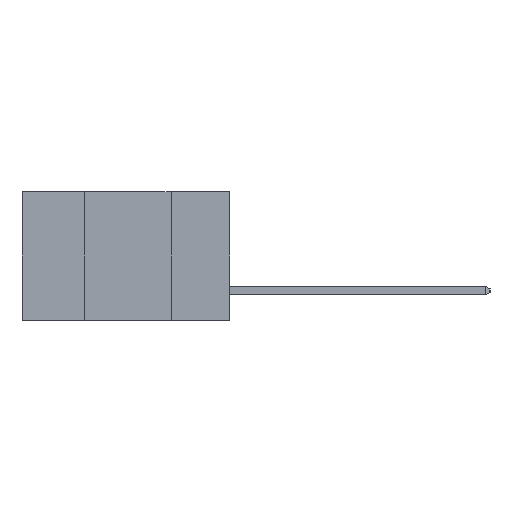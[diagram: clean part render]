
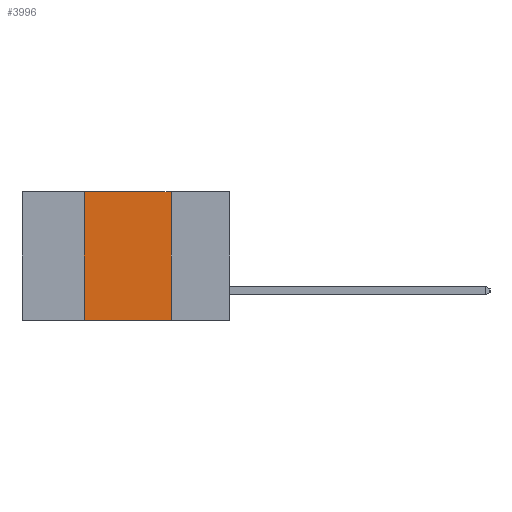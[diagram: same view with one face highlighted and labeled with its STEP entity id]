
A CAD part, left-side view. The second image highlights one B-rep face of the part: STEP entity #3996.
In plain terms, the highlighted planar face has unit normal (-1, 0, 0).
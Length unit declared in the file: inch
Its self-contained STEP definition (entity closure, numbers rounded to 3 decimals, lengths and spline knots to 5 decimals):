
#415 = CARTESIAN_POINT ( 'NONE',  ( 0., 0.42, 0. ) ) ;
#2608 = EDGE_CURVE ( 'NONE', #20251, #4977, #11109, .T. ) ;
#2613 = ORIENTED_EDGE ( 'NONE', *, *, #5116, .T. ) ;
#3695 = CARTESIAN_POINT ( 'NONE',  ( 0., 0.42, 0. ) ) ;
#3996 = ADVANCED_FACE ( 'NONE', ( #5740 ), #12449, .F. ) ;
#4363 = ORIENTED_EDGE ( 'NONE', *, *, #2608, .F. ) ;
#4509 = CARTESIAN_POINT ( 'NONE',  ( 0., 0.17, 0. ) ) ;
#4977 = VERTEX_POINT ( 'NONE', #13974 ) ;
#5116 = EDGE_CURVE ( 'NONE', #19353, #14410, #10900, .T. ) ;
#5600 = EDGE_CURVE ( 'NONE', #4977, #14410, #23228, .T. ) ;
#5740 = FACE_OUTER_BOUND ( 'NONE', #22724, .T. ) ;
#6838 = DIRECTION ( 'NONE',  ( 0., -1., 0. ) ) ;
#7258 = CARTESIAN_POINT ( 'NONE',  ( 0., 0.42, -0.37 ) ) ;
#10111 = CARTESIAN_POINT ( 'NONE',  ( 0., 0.17, -0.37 ) ) ;
#10900 = LINE ( 'NONE', #12313, #20106 ) ;
#10924 = CARTESIAN_POINT ( 'NONE',  ( 0., 0.6, 0. ) ) ;
#11091 = VECTOR ( 'NONE', #11668, 39.37008 ) ;
#11109 = LINE ( 'NONE', #10924, #15462 ) ;
#11668 = DIRECTION ( 'NONE',  ( 0., 0., 1. ) ) ;
#12313 = CARTESIAN_POINT ( 'NONE',  ( 0., 0.6, -0.37 ) ) ;
#12449 = PLANE ( 'NONE',  #22517 ) ;
#12650 = DIRECTION ( 'NONE',  ( 0., 0., -1. ) ) ;
#13214 = CARTESIAN_POINT ( 'NONE',  ( 0., 0.6, 0. ) ) ;
#13483 = VECTOR ( 'NONE', #12650, 39.37008 ) ;
#13974 = CARTESIAN_POINT ( 'NONE',  ( 0., 0.17, 0. ) ) ;
#14410 = VERTEX_POINT ( 'NONE', #10111 ) ;
#15462 = VECTOR ( 'NONE', #23221, 39.37008 ) ;
#16021 = LINE ( 'NONE', #415, #11091 ) ;
#18297 = EDGE_CURVE ( 'NONE', #19353, #20251, #16021, .T. ) ;
#19353 = VERTEX_POINT ( 'NONE', #7258 ) ;
#19949 = ORIENTED_EDGE ( 'NONE', *, *, #5600, .F. ) ;
#19973 = ORIENTED_EDGE ( 'NONE', *, *, #18297, .F. ) ;
#20106 = VECTOR ( 'NONE', #6838, 39.37008 ) ;
#20251 = VERTEX_POINT ( 'NONE', #3695 ) ;
#21408 = DIRECTION ( 'NONE',  ( 0., 0., -1. ) ) ;
#21445 = DIRECTION ( 'NONE',  ( 1., 0., 0. ) ) ;
#22517 = AXIS2_PLACEMENT_3D ( 'NONE', #13214, #21445, #21408 ) ;
#22724 = EDGE_LOOP ( 'NONE', ( #19949, #4363, #19973, #2613 ) ) ;
#23221 = DIRECTION ( 'NONE',  ( 0., -1., 0. ) ) ;
#23228 = LINE ( 'NONE', #4509, #13483 ) ;
